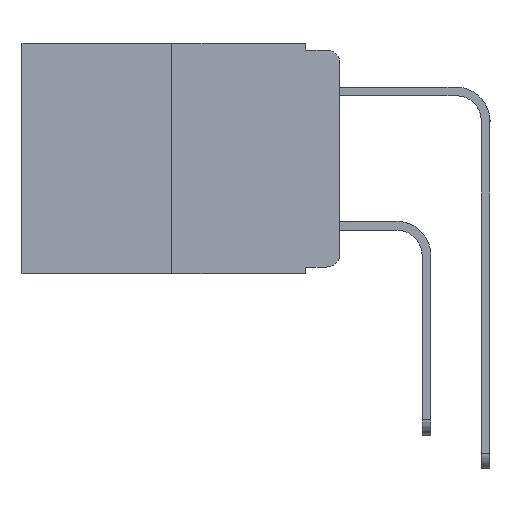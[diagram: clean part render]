
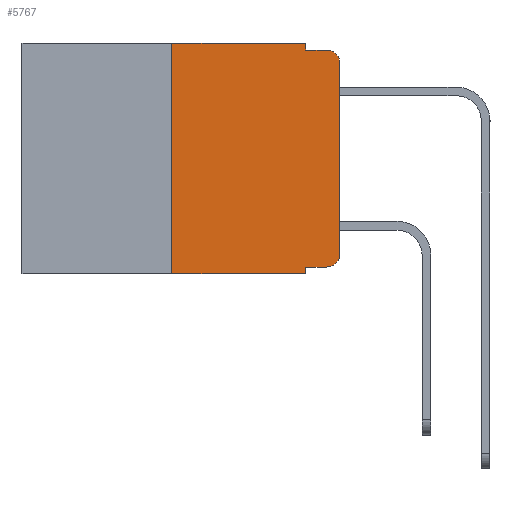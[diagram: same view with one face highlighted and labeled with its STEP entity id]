
A CAD part, left-side view. The second image highlights one B-rep face of the part: STEP entity #5767.
In plain terms, the highlighted planar face has unit normal (-1, 0, 0).
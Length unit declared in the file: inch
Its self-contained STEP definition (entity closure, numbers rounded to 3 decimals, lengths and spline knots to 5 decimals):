
#16 = EDGE_CURVE ( 'NONE', #12266, #2495, #4362, .T. ) ;
#119 = LINE ( 'NONE', #7912, #5832 ) ;
#220 = ORIENTED_EDGE ( 'NONE', *, *, #5988, .T. ) ;
#302 = EDGE_CURVE ( 'NONE', #630, #12266, #10108, .T. ) ;
#357 = CARTESIAN_POINT ( 'NONE',  ( 0., 0.051, 0. ) ) ;
#481 = VERTEX_POINT ( 'NONE', #3222 ) ;
#630 = VERTEX_POINT ( 'NONE', #357 ) ;
#1327 = CARTESIAN_POINT ( 'NONE',  ( 0., 0.051, -0.01 ) ) ;
#1475 = DIRECTION ( 'NONE',  ( 1., 0., 0. ) ) ;
#1525 = ORIENTED_EDGE ( 'NONE', *, *, #10816, .F. ) ;
#1537 = ORIENTED_EDGE ( 'NONE', *, *, #7109, .T. ) ;
#1547 = AXIS2_PLACEMENT_3D ( 'NONE', #13672, #1475, #9316 ) ;
#1565 = ORIENTED_EDGE ( 'NONE', *, *, #3089, .T. ) ;
#1701 = CARTESIAN_POINT ( 'NONE',  ( 0., 0.02, -0.313 ) ) ;
#1718 = ORIENTED_EDGE ( 'NONE', *, *, #8068, .T. ) ;
#2089 = CARTESIAN_POINT ( 'NONE',  ( 0., 0.25, 0. ) ) ;
#2273 = AXIS2_PLACEMENT_3D ( 'NONE', #12824, #6200, #13905 ) ;
#2495 = VERTEX_POINT ( 'NONE', #12956 ) ;
#2621 = LINE ( 'NONE', #4429, #11153 ) ;
#2855 = DIRECTION ( 'NONE',  ( 0., 0., -1. ) ) ;
#2894 = VECTOR ( 'NONE', #7473, 39.37008 ) ;
#2898 = DIRECTION ( 'NONE',  ( 0., 0., -1. ) ) ;
#3089 = EDGE_CURVE ( 'NONE', #481, #5131, #5858, .T. ) ;
#3222 = CARTESIAN_POINT ( 'NONE',  ( 0., 0.051, -0.333 ) ) ;
#3324 = VECTOR ( 'NONE', #7227, 39.37008 ) ;
#3433 = DIRECTION ( 'NONE',  ( 0., 0., -1. ) ) ;
#3486 = VECTOR ( 'NONE', #3433, 39.37008 ) ;
#3548 = CARTESIAN_POINT ( 'NONE',  ( 0., 0., -0.313 ) ) ;
#4045 = VERTEX_POINT ( 'NONE', #10846 ) ;
#4362 = LINE ( 'NONE', #1327, #6990 ) ;
#4429 = CARTESIAN_POINT ( 'NONE',  ( 0., 0.473, -0.343 ) ) ;
#4692 = EDGE_CURVE ( 'NONE', #4045, #9031, #119, .T. ) ;
#4820 = PLANE ( 'NONE',  #1547 ) ;
#5019 = CARTESIAN_POINT ( 'NONE',  ( 0., 0., -0.03 ) ) ;
#5106 = VECTOR ( 'NONE', #10767, 39.37008 ) ;
#5131 = VERTEX_POINT ( 'NONE', #8328 ) ;
#5204 = CARTESIAN_POINT ( 'NONE',  ( 0., 0., 0. ) ) ;
#5560 = DIRECTION ( 'NONE',  ( 0., -1., 0. ) ) ;
#5576 = ORIENTED_EDGE ( 'NONE', *, *, #8793, .F. ) ;
#5767 = ADVANCED_FACE ( 'NONE', ( #14403 ), #4820, .F. ) ;
#5832 = VECTOR ( 'NONE', #7866, 39.37008 ) ;
#5858 = LINE ( 'NONE', #10766, #2894 ) ;
#5988 = EDGE_CURVE ( 'NONE', #9919, #13923, #8426, .T. ) ;
#5989 = ORIENTED_EDGE ( 'NONE', *, *, #4692, .F. ) ;
#6200 = DIRECTION ( 'NONE',  ( -1., 0., 0. ) ) ;
#6990 = VECTOR ( 'NONE', #7652, 39.37008 ) ;
#7109 = EDGE_CURVE ( 'NONE', #5131, #9919, #12226, .T. ) ;
#7227 = DIRECTION ( 'NONE',  ( 0., -1., 0. ) ) ;
#7473 = DIRECTION ( 'NONE',  ( 0., -1., 0. ) ) ;
#7652 = DIRECTION ( 'NONE',  ( 0., -1., 0. ) ) ;
#7817 = ORIENTED_EDGE ( 'NONE', *, *, #13942, .T. ) ;
#7859 = ORIENTED_EDGE ( 'NONE', *, *, #302, .F. ) ;
#7866 = DIRECTION ( 'NONE',  ( 0., 0., 1. ) ) ;
#7912 = CARTESIAN_POINT ( 'NONE',  ( 0., 0.25, 0. ) ) ;
#8068 = EDGE_CURVE ( 'NONE', #4045, #9959, #2621, .T. ) ;
#8131 = VECTOR ( 'NONE', #2898, 39.37008 ) ;
#8328 = CARTESIAN_POINT ( 'NONE',  ( 0., 0.02, -0.333 ) ) ;
#8426 = LINE ( 'NONE', #5204, #5106 ) ;
#8767 = CIRCLE ( 'NONE', #2273, 0.02 ) ;
#8793 = EDGE_CURVE ( 'NONE', #9031, #630, #8889, .T. ) ;
#8889 = LINE ( 'NONE', #10590, #3324 ) ;
#9031 = VERTEX_POINT ( 'NONE', #2089 ) ;
#9071 = ORIENTED_EDGE ( 'NONE', *, *, #16, .F. ) ;
#9316 = DIRECTION ( 'NONE',  ( 0., 0., -1. ) ) ;
#9531 = DIRECTION ( 'NONE',  ( -1., 0., 0. ) ) ;
#9919 = VERTEX_POINT ( 'NONE', #3548 ) ;
#9959 = VERTEX_POINT ( 'NONE', #12498 ) ;
#10108 = LINE ( 'NONE', #11708, #3486 ) ;
#10590 = CARTESIAN_POINT ( 'NONE',  ( 0., 0.473, 0. ) ) ;
#10680 = CARTESIAN_POINT ( 'NONE',  ( 0., 0.051, 0. ) ) ;
#10756 = LINE ( 'NONE', #10680, #8131 ) ;
#10766 = CARTESIAN_POINT ( 'NONE',  ( 0., 0.051, -0.333 ) ) ;
#10767 = DIRECTION ( 'NONE',  ( 0., 0., 1. ) ) ;
#10816 = EDGE_CURVE ( 'NONE', #481, #9959, #10756, .T. ) ;
#10846 = CARTESIAN_POINT ( 'NONE',  ( 0., 0.25, -0.343 ) ) ;
#10855 = CARTESIAN_POINT ( 'NONE',  ( 0., 0.051, -0.01 ) ) ;
#10935 = AXIS2_PLACEMENT_3D ( 'NONE', #1701, #9531, #2855 ) ;
#11153 = VECTOR ( 'NONE', #5560, 39.37008 ) ;
#11708 = CARTESIAN_POINT ( 'NONE',  ( 0., 0.051, 0. ) ) ;
#12226 = CIRCLE ( 'NONE', #10935, 0.02 ) ;
#12266 = VERTEX_POINT ( 'NONE', #10855 ) ;
#12429 = EDGE_LOOP ( 'NONE', ( #220, #7817, #9071, #7859, #5576, #5989, #1718, #1525, #1565, #1537 ) ) ;
#12498 = CARTESIAN_POINT ( 'NONE',  ( 0., 0.051, -0.343 ) ) ;
#12824 = CARTESIAN_POINT ( 'NONE',  ( 0., 0.02, -0.03 ) ) ;
#12956 = CARTESIAN_POINT ( 'NONE',  ( 0., 0.02, -0.01 ) ) ;
#13672 = CARTESIAN_POINT ( 'NONE',  ( 0., 0.473, 0. ) ) ;
#13905 = DIRECTION ( 'NONE',  ( 0., 0., -1. ) ) ;
#13923 = VERTEX_POINT ( 'NONE', #5019 ) ;
#13942 = EDGE_CURVE ( 'NONE', #13923, #2495, #8767, .T. ) ;
#14403 = FACE_OUTER_BOUND ( 'NONE', #12429, .T. ) ;
